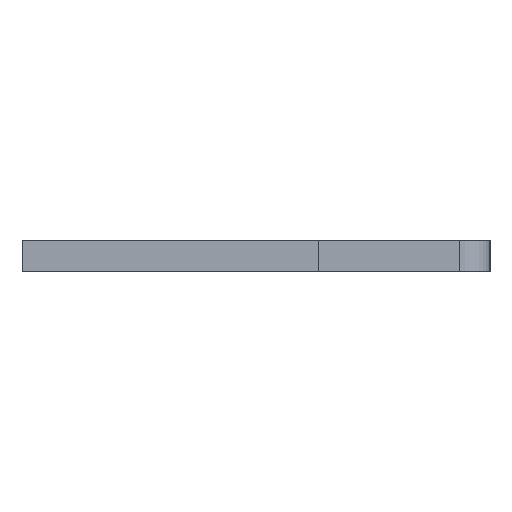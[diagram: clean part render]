
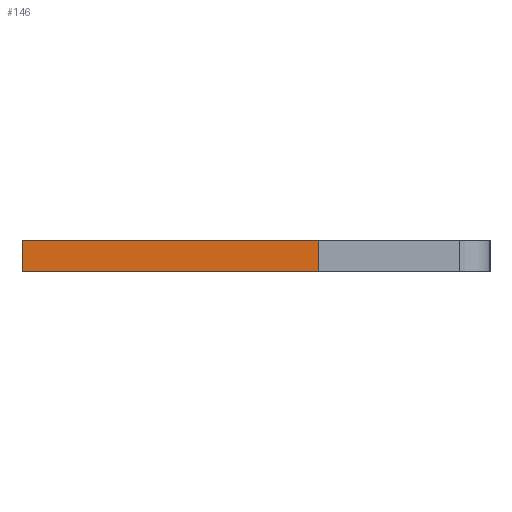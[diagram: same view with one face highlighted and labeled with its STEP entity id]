
A CAD part, left-side view. The second image highlights one B-rep face of the part: STEP entity #146.
In plain terms, the highlighted face is planar.
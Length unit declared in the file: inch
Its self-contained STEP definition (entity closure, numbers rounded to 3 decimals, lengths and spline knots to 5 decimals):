
#58 = VERTEX_POINT ( 'NONE', #482 ) ;
#90 = VECTOR ( 'NONE', #1336, 39.37008 ) ;
#127 = FACE_OUTER_BOUND ( 'NONE', #144, .T. ) ;
#144 = EDGE_LOOP ( 'NONE', ( #749, #285, #961, #238 ) ) ;
#146 = ADVANCED_FACE ( 'NONE', ( #127 ), #915, .F. ) ;
#213 = VECTOR ( 'NONE', #1188, 39.37008 ) ;
#226 = EDGE_CURVE ( 'NONE', #278, #924, #1163, .T. ) ;
#238 = ORIENTED_EDGE ( 'NONE', *, *, #824, .T. ) ;
#278 = VERTEX_POINT ( 'NONE', #955 ) ;
#285 = ORIENTED_EDGE ( 'NONE', *, *, #949, .F. ) ;
#310 = VECTOR ( 'NONE', #395, 39.37008 ) ;
#328 = DIRECTION ( 'NONE',  ( -1., 0., 0. ) ) ;
#359 = VECTOR ( 'NONE', #328, 39.37008 ) ;
#366 = DIRECTION ( 'NONE',  ( 0., 0., 1. ) ) ;
#395 = DIRECTION ( 'NONE',  ( 0., 1., 0. ) ) ;
#433 = CARTESIAN_POINT ( 'NONE',  ( -0.01, 0.15, -0.04 ) ) ;
#455 = LINE ( 'NONE', #1181, #213 ) ;
#482 = CARTESIAN_POINT ( 'NONE',  ( 0.01, 0.15, -0.04 ) ) ;
#653 = LINE ( 'NONE', #1217, #359 ) ;
#696 = DIRECTION ( 'NONE',  ( 1., 0., 0. ) ) ;
#721 = CARTESIAN_POINT ( 'NONE',  ( -0.01, 0.15, -0.04 ) ) ;
#743 = EDGE_CURVE ( 'NONE', #1157, #58, #455, .T. ) ;
#749 = ORIENTED_EDGE ( 'NONE', *, *, #226, .T. ) ;
#811 = AXIS2_PLACEMENT_3D ( 'NONE', #1260, #366, #696 ) ;
#824 = EDGE_CURVE ( 'NONE', #1157, #278, #1183, .T. ) ;
#915 = PLANE ( 'NONE',  #811 ) ;
#924 = VERTEX_POINT ( 'NONE', #433 ) ;
#949 = EDGE_CURVE ( 'NONE', #58, #924, #653, .T. ) ;
#955 = CARTESIAN_POINT ( 'NONE',  ( -0.01, -0.04, -0.04 ) ) ;
#961 = ORIENTED_EDGE ( 'NONE', *, *, #743, .F. ) ;
#1136 = CARTESIAN_POINT ( 'NONE',  ( 0.01, -0.04, -0.04 ) ) ;
#1157 = VERTEX_POINT ( 'NONE', #1136 ) ;
#1163 = LINE ( 'NONE', #721, #310 ) ;
#1181 = CARTESIAN_POINT ( 'NONE',  ( 0.01, 0.15, -0.04 ) ) ;
#1183 = LINE ( 'NONE', #1403, #90 ) ;
#1188 = DIRECTION ( 'NONE',  ( 0., 1., 0. ) ) ;
#1217 = CARTESIAN_POINT ( 'NONE',  ( 0.01, 0.15, -0.04 ) ) ;
#1260 = CARTESIAN_POINT ( 'NONE',  ( 0.01, 0.15, -0.04 ) ) ;
#1336 = DIRECTION ( 'NONE',  ( -1., 0., 0. ) ) ;
#1403 = CARTESIAN_POINT ( 'NONE',  ( 0.01, -0.04, -0.04 ) ) ;
